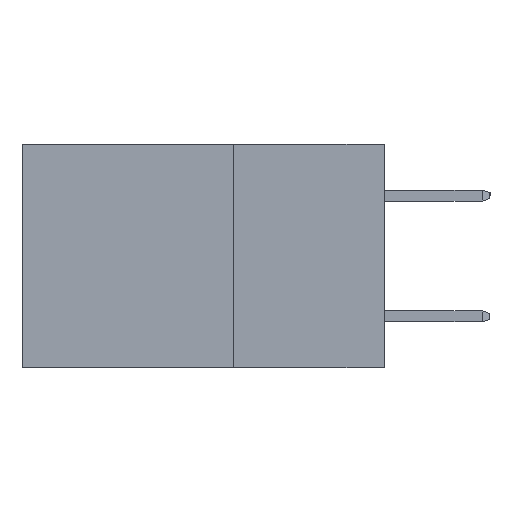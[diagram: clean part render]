
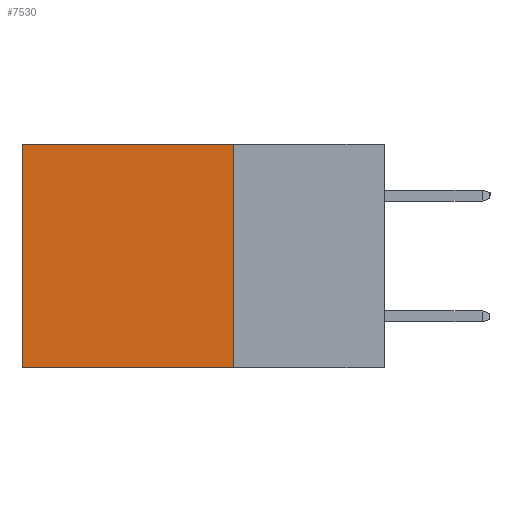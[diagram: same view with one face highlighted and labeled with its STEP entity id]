
A CAD part, left-side view. The second image highlights one B-rep face of the part: STEP entity #7530.
In plain terms, the highlighted planar face has unit normal (-1, 0, 0).
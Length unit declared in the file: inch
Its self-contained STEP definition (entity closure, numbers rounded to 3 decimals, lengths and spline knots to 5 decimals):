
#341 = ORIENTED_EDGE ( 'NONE', *, *, #16115, .T. ) ;
#732 = CARTESIAN_POINT ( 'NONE',  ( 0.2615, 0.25, 0. ) ) ;
#1030 = CARTESIAN_POINT ( 'NONE',  ( 0.2615, 0.25, -0.37 ) ) ;
#1150 = VECTOR ( 'NONE', #6411, 39.37008 ) ;
#1303 = LINE ( 'NONE', #5004, #1150 ) ;
#1667 = CARTESIAN_POINT ( 'NONE',  ( 0.2615, 0.6, -0.37 ) ) ;
#2571 = AXIS2_PLACEMENT_3D ( 'NONE', #1030, #9556, #10874 ) ;
#3482 = LINE ( 'NONE', #732, #10809 ) ;
#3631 = EDGE_CURVE ( 'NONE', #8528, #14147, #1303, .T. ) ;
#3862 = CARTESIAN_POINT ( 'NONE',  ( 0.2615, 0.6, 0. ) ) ;
#4200 = EDGE_CURVE ( 'NONE', #10580, #14147, #8362, .T. ) ;
#4252 = EDGE_LOOP ( 'NONE', ( #13942, #15045, #15820, #341 ) ) ;
#4992 = VECTOR ( 'NONE', #15358, 39.37008 ) ;
#5004 = CARTESIAN_POINT ( 'NONE',  ( 0.2615, 0.6, -0.37 ) ) ;
#5232 = VERTEX_POINT ( 'NONE', #14661 ) ;
#6411 = DIRECTION ( 'NONE',  ( 0., 0., -1. ) ) ;
#7222 = FACE_OUTER_BOUND ( 'NONE', #4252, .T. ) ;
#7530 = ADVANCED_FACE ( 'NONE', ( #7222 ), #12442, .F. ) ;
#8362 = LINE ( 'NONE', #12177, #15281 ) ;
#8528 = VERTEX_POINT ( 'NONE', #3862 ) ;
#8891 = EDGE_CURVE ( 'NONE', #5232, #10580, #16377, .T. ) ;
#9556 = DIRECTION ( 'NONE',  ( 1., 0., 0. ) ) ;
#10291 = CARTESIAN_POINT ( 'NONE',  ( 0.2615, 0.25, -0.37 ) ) ;
#10580 = VERTEX_POINT ( 'NONE', #12268 ) ;
#10809 = VECTOR ( 'NONE', #12161, 39.37008 ) ;
#10874 = DIRECTION ( 'NONE',  ( 0., 0., -1. ) ) ;
#12161 = DIRECTION ( 'NONE',  ( 0., 1., 0. ) ) ;
#12177 = CARTESIAN_POINT ( 'NONE',  ( 0.2615, 0.25, -0.37 ) ) ;
#12268 = CARTESIAN_POINT ( 'NONE',  ( 0.2615, 0.25, -0.37 ) ) ;
#12442 = PLANE ( 'NONE',  #2571 ) ;
#13942 = ORIENTED_EDGE ( 'NONE', *, *, #3631, .T. ) ;
#14147 = VERTEX_POINT ( 'NONE', #1667 ) ;
#14661 = CARTESIAN_POINT ( 'NONE',  ( 0.2615, 0.25, 0. ) ) ;
#15045 = ORIENTED_EDGE ( 'NONE', *, *, #4200, .F. ) ;
#15281 = VECTOR ( 'NONE', #15766, 39.37008 ) ;
#15358 = DIRECTION ( 'NONE',  ( 0., 0., -1. ) ) ;
#15766 = DIRECTION ( 'NONE',  ( 0., 1., 0. ) ) ;
#15820 = ORIENTED_EDGE ( 'NONE', *, *, #8891, .F. ) ;
#16115 = EDGE_CURVE ( 'NONE', #5232, #8528, #3482, .T. ) ;
#16377 = LINE ( 'NONE', #10291, #4992 ) ;
